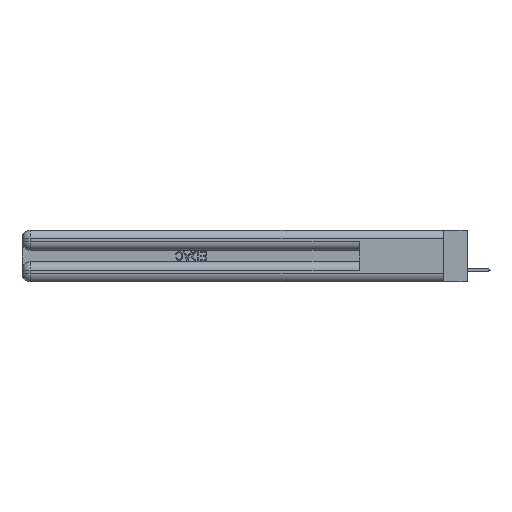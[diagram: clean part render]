
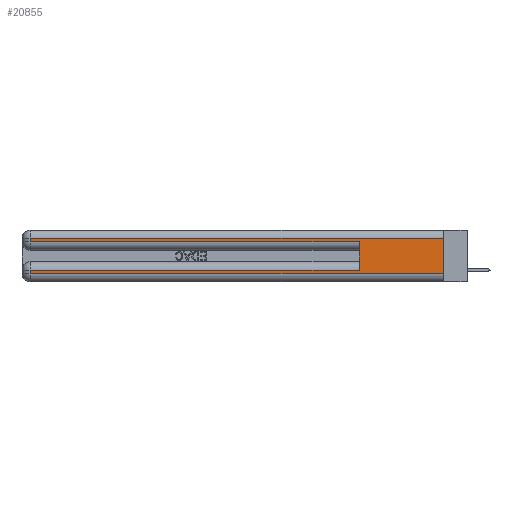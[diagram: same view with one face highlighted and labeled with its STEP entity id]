
A CAD part, left-side view. The second image highlights one B-rep face of the part: STEP entity #20855.
In plain terms, the highlighted planar face has unit normal (-1, 0, 0).
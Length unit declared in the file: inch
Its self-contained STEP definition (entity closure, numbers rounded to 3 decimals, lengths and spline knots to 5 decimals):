
#15 = VECTOR ( 'NONE', #6484, 39.37008 ) ;
#361 = DIRECTION ( 'NONE',  ( 0., -1., 0. ) ) ;
#1020 = EDGE_LOOP ( 'NONE', ( #13116, #24633, #27897, #43274, #32824, #26891, #7148, #38572 ) ) ;
#1430 = VECTOR ( 'NONE', #36964, 39.37008 ) ;
#1535 = DIRECTION ( 'NONE',  ( 0., -1., 0. ) ) ;
#2234 = CARTESIAN_POINT ( 'NONE',  ( 0., 2.94, 0.06 ) ) ;
#2637 = VERTEX_POINT ( 'NONE', #19274 ) ;
#2789 = EDGE_CURVE ( 'NONE', #20303, #13259, #28446, .T. ) ;
#5574 = VECTOR ( 'NONE', #37635, 39.37008 ) ;
#5618 = EDGE_CURVE ( 'NONE', #2637, #17624, #38972, .T. ) ;
#5734 = FACE_OUTER_BOUND ( 'NONE', #1020, .T. ) ;
#6269 = LINE ( 'NONE', #28411, #43212 ) ;
#6298 = EDGE_CURVE ( 'NONE', #28113, #27150, #6269, .T. ) ;
#6484 = DIRECTION ( 'NONE',  ( 0., 0., -1. ) ) ;
#7148 = ORIENTED_EDGE ( 'NONE', *, *, #37206, .T. ) ;
#7951 = VERTEX_POINT ( 'NONE', #16765 ) ;
#8669 = AXIS2_PLACEMENT_3D ( 'NONE', #15822, #32394, #39738 ) ;
#9718 = VECTOR ( 'NONE', #32692, 39.37008 ) ;
#11767 = PLANE ( 'NONE',  #8669 ) ;
#13116 = ORIENTED_EDGE ( 'NONE', *, *, #41542, .F. ) ;
#13259 = VERTEX_POINT ( 'NONE', #14546 ) ;
#13426 = CARTESIAN_POINT ( 'NONE',  ( 0., 2.94, 0.37 ) ) ;
#14546 = CARTESIAN_POINT ( 'NONE',  ( 0., 2.94, 0.31 ) ) ;
#14721 = LINE ( 'NONE', #30764, #5574 ) ;
#15044 = CARTESIAN_POINT ( 'NONE',  ( 0., 2.94, 0.085 ) ) ;
#15822 = CARTESIAN_POINT ( 'NONE',  ( 0., 0., 0.37 ) ) ;
#16765 = CARTESIAN_POINT ( 'NONE',  ( 0., 2.94, 0.285 ) ) ;
#17624 = VERTEX_POINT ( 'NONE', #33792 ) ;
#17867 = CARTESIAN_POINT ( 'NONE',  ( 0., 0., 0.285 ) ) ;
#19274 = CARTESIAN_POINT ( 'NONE',  ( 0., 0.6, 0.085 ) ) ;
#19629 = VECTOR ( 'NONE', #361, 39.37008 ) ;
#20103 = CARTESIAN_POINT ( 'NONE',  ( 0., 0.6, 0.145 ) ) ;
#20227 = CARTESIAN_POINT ( 'NONE',  ( 0., 0., 0.06 ) ) ;
#20303 = VERTEX_POINT ( 'NONE', #25605 ) ;
#20855 = ADVANCED_FACE ( 'NONE', ( #5734 ), #11767, .F. ) ;
#22521 = VERTEX_POINT ( 'NONE', #15044 ) ;
#24126 = CARTESIAN_POINT ( 'NONE',  ( 0., 2.94, 0.37 ) ) ;
#24155 = CARTESIAN_POINT ( 'NONE',  ( 0., 0., 0.31 ) ) ;
#24633 = ORIENTED_EDGE ( 'NONE', *, *, #2789, .T. ) ;
#25605 = CARTESIAN_POINT ( 'NONE',  ( 0., 0., 0.31 ) ) ;
#26573 = LINE ( 'NONE', #17867, #19629 ) ;
#26599 = CARTESIAN_POINT ( 'NONE',  ( 0., 0., 0.37 ) ) ;
#26891 = ORIENTED_EDGE ( 'NONE', *, *, #27951, .T. ) ;
#27150 = VERTEX_POINT ( 'NONE', #20227 ) ;
#27897 = ORIENTED_EDGE ( 'NONE', *, *, #34764, .T. ) ;
#27951 = EDGE_CURVE ( 'NONE', #2637, #22521, #14721, .T. ) ;
#28113 = VERTEX_POINT ( 'NONE', #2234 ) ;
#28411 = CARTESIAN_POINT ( 'NONE',  ( 0., 0., 0.06 ) ) ;
#28446 = LINE ( 'NONE', #24155, #9718 ) ;
#30764 = CARTESIAN_POINT ( 'NONE',  ( 0., 0., 0.085 ) ) ;
#31633 = VECTOR ( 'NONE', #36650, 39.37008 ) ;
#32394 = DIRECTION ( 'NONE',  ( 1., 0., 0. ) ) ;
#32505 = EDGE_CURVE ( 'NONE', #7951, #17624, #26573, .T. ) ;
#32692 = DIRECTION ( 'NONE',  ( 0., 1., 0. ) ) ;
#32824 = ORIENTED_EDGE ( 'NONE', *, *, #5618, .F. ) ;
#33062 = VECTOR ( 'NONE', #38181, 39.37008 ) ;
#33282 = LINE ( 'NONE', #13426, #15 ) ;
#33792 = CARTESIAN_POINT ( 'NONE',  ( 0., 0.6, 0.285 ) ) ;
#34764 = EDGE_CURVE ( 'NONE', #13259, #7951, #33282, .T. ) ;
#36650 = DIRECTION ( 'NONE',  ( 0., 0., -1. ) ) ;
#36964 = DIRECTION ( 'NONE',  ( 0., 0., 1. ) ) ;
#37206 = EDGE_CURVE ( 'NONE', #22521, #28113, #42714, .T. ) ;
#37635 = DIRECTION ( 'NONE',  ( 0., 1., 0. ) ) ;
#38181 = DIRECTION ( 'NONE',  ( 0., 0., -1. ) ) ;
#38572 = ORIENTED_EDGE ( 'NONE', *, *, #6298, .T. ) ;
#38972 = LINE ( 'NONE', #20103, #1430 ) ;
#39738 = DIRECTION ( 'NONE',  ( 0., 0., -1. ) ) ;
#41542 = EDGE_CURVE ( 'NONE', #20303, #27150, #43993, .T. ) ;
#42714 = LINE ( 'NONE', #24126, #33062 ) ;
#43212 = VECTOR ( 'NONE', #1535, 39.37008 ) ;
#43274 = ORIENTED_EDGE ( 'NONE', *, *, #32505, .T. ) ;
#43993 = LINE ( 'NONE', #26599, #31633 ) ;
